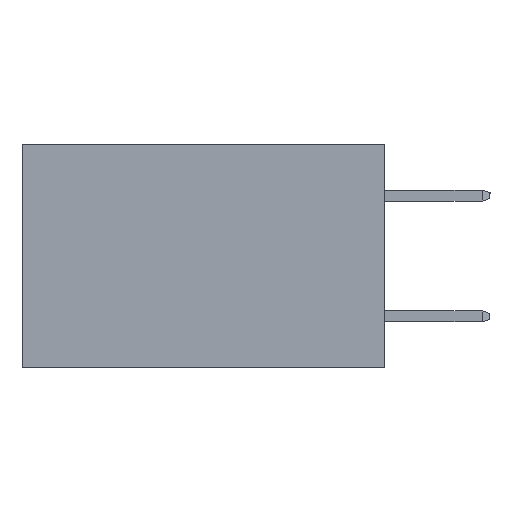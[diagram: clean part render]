
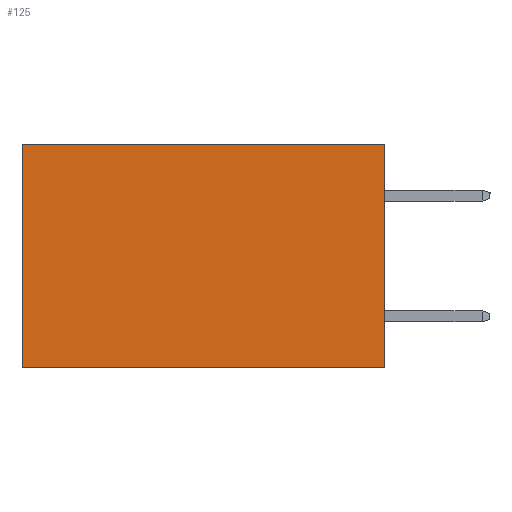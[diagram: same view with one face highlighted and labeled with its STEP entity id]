
A CAD part, left-side view. The second image highlights one B-rep face of the part: STEP entity #125.
In plain terms, the highlighted planar face has unit normal (-1, 0, 0).
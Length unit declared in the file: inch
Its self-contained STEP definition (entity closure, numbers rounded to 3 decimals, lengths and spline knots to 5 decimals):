
#125 = ADVANCED_FACE ( 'NONE', ( #14769 ), #3253, .F. ) ;
#390 = LINE ( 'NONE', #1639, #9279 ) ;
#1628 = VERTEX_POINT ( 'NONE', #16354 ) ;
#1639 = CARTESIAN_POINT ( 'NONE',  ( 0.2615, 0., -0.37 ) ) ;
#2250 = EDGE_CURVE ( 'NONE', #1628, #8380, #10159, .T. ) ;
#2489 = DIRECTION ( 'NONE',  ( 0., 0., -1. ) ) ;
#2776 = AXIS2_PLACEMENT_3D ( 'NONE', #13511, #5851, #10962 ) ;
#3253 = PLANE ( 'NONE',  #2776 ) ;
#3528 = ORIENTED_EDGE ( 'NONE', *, *, #7629, .F. ) ;
#5230 = VECTOR ( 'NONE', #10579, 39.37008 ) ;
#5268 = DIRECTION ( 'NONE',  ( 0., 0., -1. ) ) ;
#5693 = ORIENTED_EDGE ( 'NONE', *, *, #2250, .F. ) ;
#5851 = DIRECTION ( 'NONE',  ( 1., 0., 0. ) ) ;
#6026 = VECTOR ( 'NONE', #2489, 39.37008 ) ;
#6423 = CARTESIAN_POINT ( 'NONE',  ( 0.2615, 0., -0.37 ) ) ;
#6658 = VERTEX_POINT ( 'NONE', #12209 ) ;
#6671 = EDGE_CURVE ( 'NONE', #1628, #6658, #16013, .T. ) ;
#6718 = CARTESIAN_POINT ( 'NONE',  ( 0.2615, 0., 0. ) ) ;
#6727 = DIRECTION ( 'NONE',  ( 0., 1., 0. ) ) ;
#7629 = EDGE_CURVE ( 'NONE', #8380, #14731, #390, .T. ) ;
#8380 = VERTEX_POINT ( 'NONE', #15865 ) ;
#8664 = EDGE_CURVE ( 'NONE', #6658, #14731, #11466, .T. ) ;
#9140 = VECTOR ( 'NONE', #5268, 39.37008 ) ;
#9279 = VECTOR ( 'NONE', #6727, 39.37008 ) ;
#10159 = LINE ( 'NONE', #6423, #9140 ) ;
#10579 = DIRECTION ( 'NONE',  ( 0., 1., 0. ) ) ;
#10962 = DIRECTION ( 'NONE',  ( 0., 0., -1. ) ) ;
#11466 = LINE ( 'NONE', #14149, #6026 ) ;
#12002 = CARTESIAN_POINT ( 'NONE',  ( 0.2615, 0.6, -0.37 ) ) ;
#12209 = CARTESIAN_POINT ( 'NONE',  ( 0.2615, 0.6, 0. ) ) ;
#12972 = ORIENTED_EDGE ( 'NONE', *, *, #6671, .T. ) ;
#13511 = CARTESIAN_POINT ( 'NONE',  ( 0.2615, 0., -0.37 ) ) ;
#14149 = CARTESIAN_POINT ( 'NONE',  ( 0.2615, 0.6, -0.37 ) ) ;
#14372 = ORIENTED_EDGE ( 'NONE', *, *, #8664, .T. ) ;
#14731 = VERTEX_POINT ( 'NONE', #12002 ) ;
#14769 = FACE_OUTER_BOUND ( 'NONE', #16156, .T. ) ;
#15865 = CARTESIAN_POINT ( 'NONE',  ( 0.2615, 0., -0.37 ) ) ;
#16013 = LINE ( 'NONE', #6718, #5230 ) ;
#16156 = EDGE_LOOP ( 'NONE', ( #14372, #3528, #5693, #12972 ) ) ;
#16354 = CARTESIAN_POINT ( 'NONE',  ( 0.2615, 0., 0. ) ) ;
